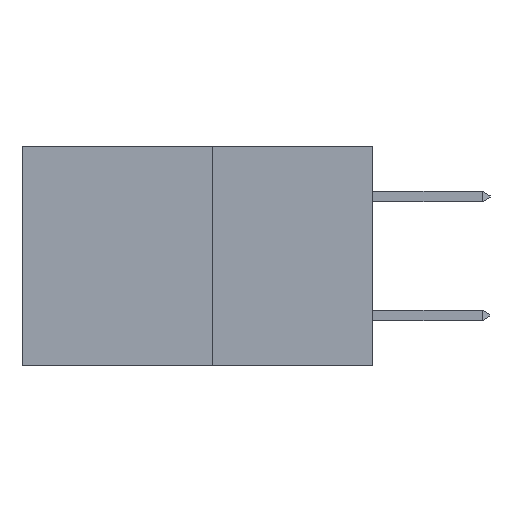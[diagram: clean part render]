
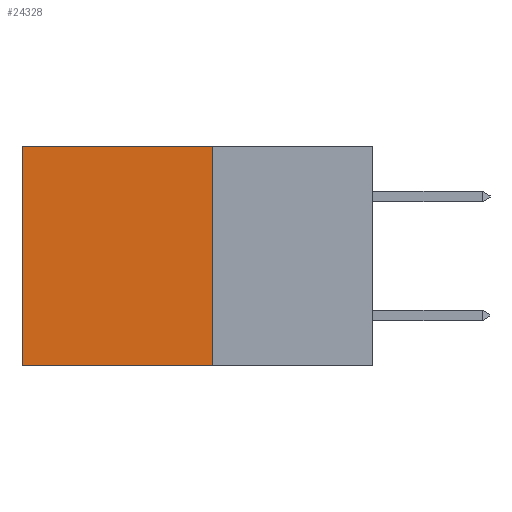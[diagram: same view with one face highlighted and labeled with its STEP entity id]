
A CAD part, left-side view. The second image highlights one B-rep face of the part: STEP entity #24328.
In plain terms, the highlighted planar face has unit normal (-1, 0, 0).
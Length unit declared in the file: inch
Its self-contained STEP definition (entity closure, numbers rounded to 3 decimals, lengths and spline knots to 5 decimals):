
#396 = ORIENTED_EDGE ( 'NONE', *, *, #11018, .F. ) ;
#595 = CARTESIAN_POINT ( 'NONE',  ( 0.277, 0.27, 0. ) ) ;
#670 = LINE ( 'NONE', #25775, #24985 ) ;
#1124 = LINE ( 'NONE', #595, #19811 ) ;
#2586 = EDGE_CURVE ( 'NONE', #19543, #12734, #670, .T. ) ;
#3349 = CARTESIAN_POINT ( 'NONE',  ( 0.277, 0.27, 0. ) ) ;
#3432 = CARTESIAN_POINT ( 'NONE',  ( 0.277, 0.59, -0.37 ) ) ;
#4365 = ORIENTED_EDGE ( 'NONE', *, *, #29549, .T. ) ;
#4898 = CARTESIAN_POINT ( 'NONE',  ( 0.277, 0.27, -0.37 ) ) ;
#5881 = DIRECTION ( 'NONE',  ( 0., 0., -1. ) ) ;
#10267 = FACE_OUTER_BOUND ( 'NONE', #20420, .T. ) ;
#10885 = PLANE ( 'NONE',  #27777 ) ;
#11018 = EDGE_CURVE ( 'NONE', #12734, #30357, #15360, .T. ) ;
#12191 = CARTESIAN_POINT ( 'NONE',  ( 0.277, 0.59, 0. ) ) ;
#12734 = VERTEX_POINT ( 'NONE', #30927 ) ;
#13323 = CARTESIAN_POINT ( 'NONE',  ( 0.277, 0.27, -0.37 ) ) ;
#15223 = DIRECTION ( 'NONE',  ( 0., 1., 0. ) ) ;
#15360 = LINE ( 'NONE', #4898, #16132 ) ;
#15599 = EDGE_CURVE ( 'NONE', #16728, #30357, #23673, .T. ) ;
#15790 = DIRECTION ( 'NONE',  ( 0., 0., -1. ) ) ;
#16132 = VECTOR ( 'NONE', #15223, 39.37008 ) ;
#16265 = ORIENTED_EDGE ( 'NONE', *, *, #15599, .T. ) ;
#16728 = VERTEX_POINT ( 'NONE', #12191 ) ;
#17266 = VECTOR ( 'NONE', #5881, 39.37008 ) ;
#19543 = VERTEX_POINT ( 'NONE', #3349 ) ;
#19811 = VECTOR ( 'NONE', #24802, 39.37008 ) ;
#20420 = EDGE_LOOP ( 'NONE', ( #16265, #396, #21633, #4365 ) ) ;
#21633 = ORIENTED_EDGE ( 'NONE', *, *, #2586, .F. ) ;
#23673 = LINE ( 'NONE', #3432, #17266 ) ;
#24328 = ADVANCED_FACE ( 'NONE', ( #10267 ), #10885, .F. ) ;
#24802 = DIRECTION ( 'NONE',  ( 0., 1., 0. ) ) ;
#24844 = DIRECTION ( 'NONE',  ( 0., 0., -1. ) ) ;
#24985 = VECTOR ( 'NONE', #24844, 39.37008 ) ;
#25775 = CARTESIAN_POINT ( 'NONE',  ( 0.277, 0.27, -0.37 ) ) ;
#27777 = AXIS2_PLACEMENT_3D ( 'NONE', #13323, #29971, #15790 ) ;
#29549 = EDGE_CURVE ( 'NONE', #19543, #16728, #1124, .T. ) ;
#29938 = CARTESIAN_POINT ( 'NONE',  ( 0.277, 0.59, -0.37 ) ) ;
#29971 = DIRECTION ( 'NONE',  ( 1., 0., 0. ) ) ;
#30357 = VERTEX_POINT ( 'NONE', #29938 ) ;
#30927 = CARTESIAN_POINT ( 'NONE',  ( 0.277, 0.27, -0.37 ) ) ;
